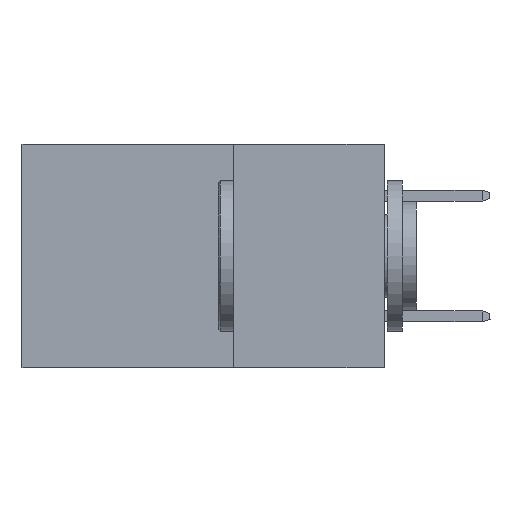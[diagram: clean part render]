
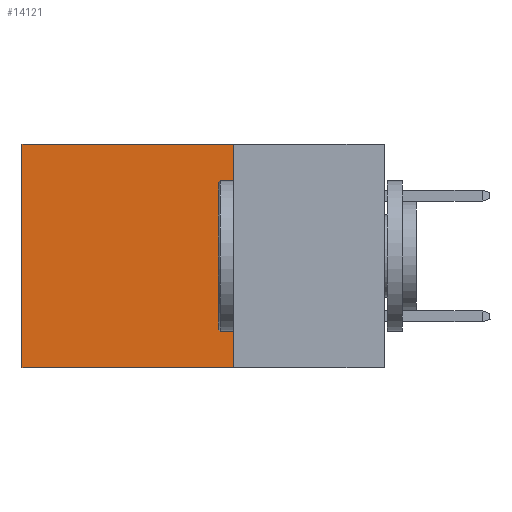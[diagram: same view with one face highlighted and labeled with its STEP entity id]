
A CAD part, left-side view. The second image highlights one B-rep face of the part: STEP entity #14121.
In plain terms, the highlighted planar face has unit normal (-1, 0, 0).
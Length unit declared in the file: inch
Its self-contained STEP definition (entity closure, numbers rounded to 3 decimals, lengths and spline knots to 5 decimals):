
#478 = DIRECTION ( 'NONE',  ( 0., 0., -1. ) ) ;
#771 = CARTESIAN_POINT ( 'NONE',  ( 0.2615, 0.6, -0.37 ) ) ;
#1269 = LINE ( 'NONE', #10798, #16445 ) ;
#2029 = ORIENTED_EDGE ( 'NONE', *, *, #3896, .T. ) ;
#2206 = VERTEX_POINT ( 'NONE', #771 ) ;
#3396 = VECTOR ( 'NONE', #4747, 39.37008 ) ;
#3896 = EDGE_CURVE ( 'NONE', #10498, #5872, #1269, .T. ) ;
#4694 = EDGE_CURVE ( 'NONE', #5872, #2206, #10385, .T. ) ;
#4747 = DIRECTION ( 'NONE',  ( 0., 1., 0. ) ) ;
#5237 = CARTESIAN_POINT ( 'NONE',  ( 0.2615, 0.6, -0.37 ) ) ;
#5251 = DIRECTION ( 'NONE',  ( 0., 0., -1. ) ) ;
#5300 = LINE ( 'NONE', #7413, #15922 ) ;
#5647 = FACE_OUTER_BOUND ( 'NONE', #7637, .T. ) ;
#5872 = VERTEX_POINT ( 'NONE', #6875 ) ;
#6875 = CARTESIAN_POINT ( 'NONE',  ( 0.2615, 0.6, 0. ) ) ;
#6979 = EDGE_CURVE ( 'NONE', #10498, #17502, #5300, .T. ) ;
#7110 = AXIS2_PLACEMENT_3D ( 'NONE', #7390, #8812, #478 ) ;
#7388 = DIRECTION ( 'NONE',  ( 0., 0., -1. ) ) ;
#7390 = CARTESIAN_POINT ( 'NONE',  ( 0.2615, 0.25, -0.37 ) ) ;
#7413 = CARTESIAN_POINT ( 'NONE',  ( 0.2615, 0.25, -0.37 ) ) ;
#7449 = PLANE ( 'NONE',  #7110 ) ;
#7637 = EDGE_LOOP ( 'NONE', ( #17318, #16905, #17902, #2029 ) ) ;
#8812 = DIRECTION ( 'NONE',  ( 1., 0., 0. ) ) ;
#10329 = EDGE_CURVE ( 'NONE', #17502, #2206, #10337, .T. ) ;
#10337 = LINE ( 'NONE', #13113, #3396 ) ;
#10385 = LINE ( 'NONE', #5237, #17691 ) ;
#10498 = VERTEX_POINT ( 'NONE', #13395 ) ;
#10798 = CARTESIAN_POINT ( 'NONE',  ( 0.2615, 0.25, 0. ) ) ;
#10991 = CARTESIAN_POINT ( 'NONE',  ( 0.2615, 0.25, -0.37 ) ) ;
#11100 = DIRECTION ( 'NONE',  ( 0., 1., 0. ) ) ;
#13113 = CARTESIAN_POINT ( 'NONE',  ( 0.2615, 0.25, -0.37 ) ) ;
#13395 = CARTESIAN_POINT ( 'NONE',  ( 0.2615, 0.25, 0. ) ) ;
#14121 = ADVANCED_FACE ( 'NONE', ( #5647 ), #7449, .F. ) ;
#15922 = VECTOR ( 'NONE', #7388, 39.37008 ) ;
#16445 = VECTOR ( 'NONE', #11100, 39.37008 ) ;
#16905 = ORIENTED_EDGE ( 'NONE', *, *, #10329, .F. ) ;
#17318 = ORIENTED_EDGE ( 'NONE', *, *, #4694, .T. ) ;
#17502 = VERTEX_POINT ( 'NONE', #10991 ) ;
#17691 = VECTOR ( 'NONE', #5251, 39.37008 ) ;
#17902 = ORIENTED_EDGE ( 'NONE', *, *, #6979, .F. ) ;
